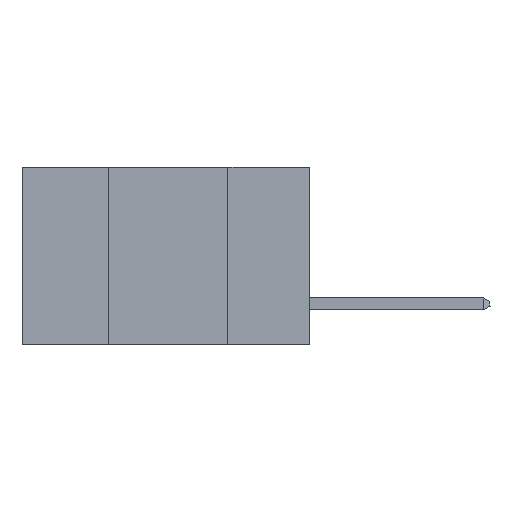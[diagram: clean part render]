
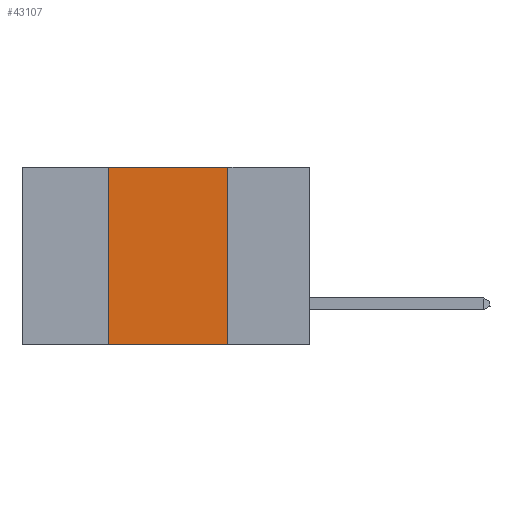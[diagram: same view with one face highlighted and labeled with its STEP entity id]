
A CAD part, left-side view. The second image highlights one B-rep face of the part: STEP entity #43107.
In plain terms, the highlighted planar face has unit normal (-1, 0, 0).
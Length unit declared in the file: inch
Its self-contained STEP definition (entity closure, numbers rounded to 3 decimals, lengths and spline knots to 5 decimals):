
#1297 = LINE ( 'NONE', #8854, #36943 ) ;
#2402 = DIRECTION ( 'NONE',  ( 1., 0., 0. ) ) ;
#4493 = VERTEX_POINT ( 'NONE', #48263 ) ;
#5983 = ORIENTED_EDGE ( 'NONE', *, *, #48855, .F. ) ;
#6604 = EDGE_CURVE ( 'NONE', #4493, #50662, #1297, .T. ) ;
#8854 = CARTESIAN_POINT ( 'NONE',  ( 0., 0.6, -0.37 ) ) ;
#11730 = CARTESIAN_POINT ( 'NONE',  ( 0., 0.17, 0. ) ) ;
#12293 = VECTOR ( 'NONE', #45518, 39.37008 ) ;
#12519 = ORIENTED_EDGE ( 'NONE', *, *, #13787, .F. ) ;
#13044 = DIRECTION ( 'NONE',  ( 0., -1., 0. ) ) ;
#13116 = CARTESIAN_POINT ( 'NONE',  ( 0., 0.42, 0. ) ) ;
#13787 = EDGE_CURVE ( 'NONE', #32704, #50662, #25229, .T. ) ;
#14972 = ORIENTED_EDGE ( 'NONE', *, *, #6604, .T. ) ;
#16130 = CARTESIAN_POINT ( 'NONE',  ( 0., 0.17, 0. ) ) ;
#18359 = DIRECTION ( 'NONE',  ( 0., 0., -1. ) ) ;
#20290 = LINE ( 'NONE', #33659, #12293 ) ;
#20873 = DIRECTION ( 'NONE',  ( 0., -1., 0. ) ) ;
#25229 = LINE ( 'NONE', #16130, #48612 ) ;
#25885 = PLANE ( 'NONE',  #37641 ) ;
#26426 = LINE ( 'NONE', #36391, #46110 ) ;
#29172 = EDGE_CURVE ( 'NONE', #43492, #32704, #26426, .T. ) ;
#32704 = VERTEX_POINT ( 'NONE', #11730 ) ;
#33659 = CARTESIAN_POINT ( 'NONE',  ( 0., 0.42, 0. ) ) ;
#34174 = CARTESIAN_POINT ( 'NONE',  ( 0., 0.6, 0. ) ) ;
#36391 = CARTESIAN_POINT ( 'NONE',  ( 0., 0.6, 0. ) ) ;
#36870 = CARTESIAN_POINT ( 'NONE',  ( 0., 0.17, -0.37 ) ) ;
#36943 = VECTOR ( 'NONE', #20873, 39.37008 ) ;
#37641 = AXIS2_PLACEMENT_3D ( 'NONE', #34174, #2402, #18359 ) ;
#39829 = DIRECTION ( 'NONE',  ( 0., 0., -1. ) ) ;
#41689 = EDGE_LOOP ( 'NONE', ( #12519, #44896, #5983, #14972 ) ) ;
#43107 = ADVANCED_FACE ( 'NONE', ( #46008 ), #25885, .F. ) ;
#43492 = VERTEX_POINT ( 'NONE', #13116 ) ;
#44896 = ORIENTED_EDGE ( 'NONE', *, *, #29172, .F. ) ;
#45518 = DIRECTION ( 'NONE',  ( 0., 0., 1. ) ) ;
#46008 = FACE_OUTER_BOUND ( 'NONE', #41689, .T. ) ;
#46110 = VECTOR ( 'NONE', #13044, 39.37008 ) ;
#48263 = CARTESIAN_POINT ( 'NONE',  ( 0., 0.42, -0.37 ) ) ;
#48612 = VECTOR ( 'NONE', #39829, 39.37008 ) ;
#48855 = EDGE_CURVE ( 'NONE', #4493, #43492, #20290, .T. ) ;
#50662 = VERTEX_POINT ( 'NONE', #36870 ) ;
